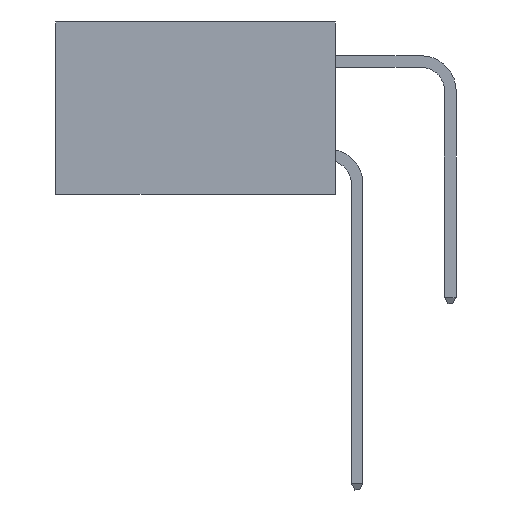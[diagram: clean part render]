
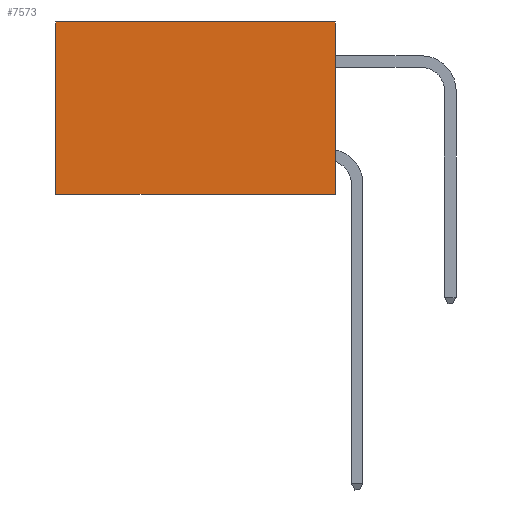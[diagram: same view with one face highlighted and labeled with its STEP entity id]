
A CAD part, left-side view. The second image highlights one B-rep face of the part: STEP entity #7573.
In plain terms, the highlighted planar face has unit normal (-1, 0, 0).
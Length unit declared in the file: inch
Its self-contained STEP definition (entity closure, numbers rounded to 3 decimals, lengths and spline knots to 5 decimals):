
#116 = VERTEX_POINT ( 'NONE', #11900 ) ;
#1093 = CARTESIAN_POINT ( 'NONE',  ( 0.2875, 0.6, 0. ) ) ;
#1163 = ORIENTED_EDGE ( 'NONE', *, *, #23906, .T. ) ;
#1696 = DIRECTION ( 'NONE',  ( 0., 0., -1. ) ) ;
#1770 = AXIS2_PLACEMENT_3D ( 'NONE', #19797, #21715, #10186 ) ;
#1873 = ORIENTED_EDGE ( 'NONE', *, *, #23298, .T. ) ;
#3364 = VECTOR ( 'NONE', #1696, 39.37008 ) ;
#3915 = DIRECTION ( 'NONE',  ( 0., 1., 0. ) ) ;
#4008 = LINE ( 'NONE', #5655, #3364 ) ;
#5655 = CARTESIAN_POINT ( 'NONE',  ( 0.2875, 0.6, 0. ) ) ;
#5725 = VERTEX_POINT ( 'NONE', #22743 ) ;
#6832 = FACE_OUTER_BOUND ( 'NONE', #13973, .T. ) ;
#7048 = CARTESIAN_POINT ( 'NONE',  ( 0.2875, 0., -0.37 ) ) ;
#7573 = ADVANCED_FACE ( 'NONE', ( #6832 ), #13994, .F. ) ;
#7824 = ORIENTED_EDGE ( 'NONE', *, *, #12694, .F. ) ;
#10111 = VECTOR ( 'NONE', #3915, 39.37008 ) ;
#10186 = DIRECTION ( 'NONE',  ( 0., 0., -1. ) ) ;
#10697 = LINE ( 'NONE', #13627, #10111 ) ;
#11467 = CARTESIAN_POINT ( 'NONE',  ( 0.2875, 0., -0.37 ) ) ;
#11900 = CARTESIAN_POINT ( 'NONE',  ( 0.2875, 0.6, -0.37 ) ) ;
#12488 = EDGE_CURVE ( 'NONE', #21798, #116, #20210, .T. ) ;
#12694 = EDGE_CURVE ( 'NONE', #5725, #21798, #20494, .T. ) ;
#13431 = DIRECTION ( 'NONE',  ( 0., 1., 0. ) ) ;
#13627 = CARTESIAN_POINT ( 'NONE',  ( 0.2875, 0., 0. ) ) ;
#13768 = ORIENTED_EDGE ( 'NONE', *, *, #12488, .F. ) ;
#13973 = EDGE_LOOP ( 'NONE', ( #1873, #13768, #7824, #1163 ) ) ;
#13994 = PLANE ( 'NONE',  #1770 ) ;
#14781 = VECTOR ( 'NONE', #21577, 39.37008 ) ;
#15731 = VECTOR ( 'NONE', #13431, 39.37008 ) ;
#18239 = VERTEX_POINT ( 'NONE', #1093 ) ;
#19797 = CARTESIAN_POINT ( 'NONE',  ( 0.2875, 0., 0. ) ) ;
#20210 = LINE ( 'NONE', #11467, #15731 ) ;
#20494 = LINE ( 'NONE', #21496, #14781 ) ;
#21496 = CARTESIAN_POINT ( 'NONE',  ( 0.2875, 0., 0. ) ) ;
#21577 = DIRECTION ( 'NONE',  ( 0., 0., -1. ) ) ;
#21715 = DIRECTION ( 'NONE',  ( 1., 0., 0. ) ) ;
#21798 = VERTEX_POINT ( 'NONE', #7048 ) ;
#22743 = CARTESIAN_POINT ( 'NONE',  ( 0.2875, 0., 0. ) ) ;
#23298 = EDGE_CURVE ( 'NONE', #18239, #116, #4008, .T. ) ;
#23906 = EDGE_CURVE ( 'NONE', #5725, #18239, #10697, .T. ) ;
